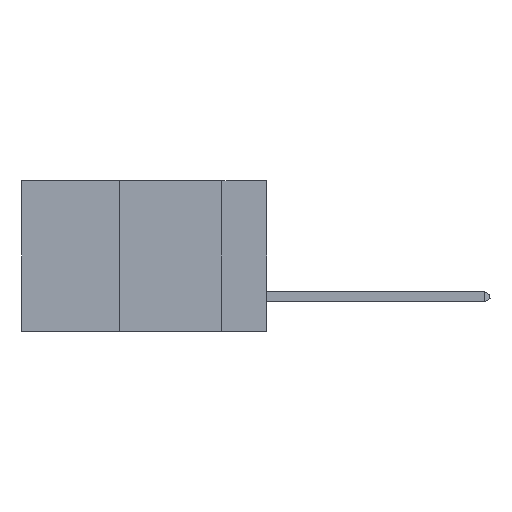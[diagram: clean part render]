
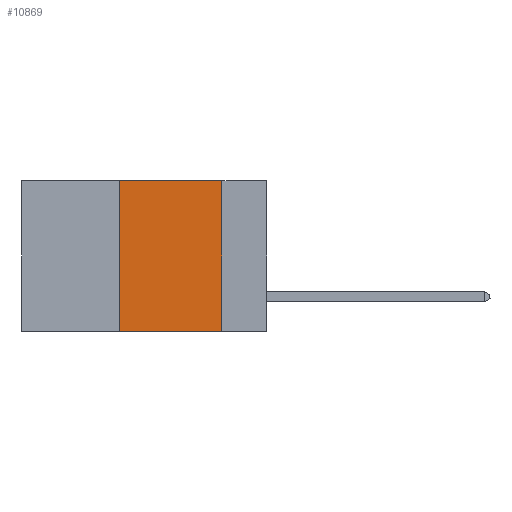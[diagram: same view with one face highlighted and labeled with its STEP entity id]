
A CAD part, left-side view. The second image highlights one B-rep face of the part: STEP entity #10869.
In plain terms, the highlighted planar face has unit normal (-1, 0, 0).
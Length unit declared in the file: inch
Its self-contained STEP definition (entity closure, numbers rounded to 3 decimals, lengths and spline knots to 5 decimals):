
#1000 = CARTESIAN_POINT ( 'NONE',  ( 0., 0.11, 0. ) ) ;
#1123 = CARTESIAN_POINT ( 'NONE',  ( 0., 0.11, -0.37 ) ) ;
#1631 = VERTEX_POINT ( 'NONE', #13952 ) ;
#2370 = DIRECTION ( 'NONE',  ( 0., 0., -1. ) ) ;
#3438 = ORIENTED_EDGE ( 'NONE', *, *, #17596, .F. ) ;
#3608 = AXIS2_PLACEMENT_3D ( 'NONE', #14501, #11351, #2370 ) ;
#3938 = LINE ( 'NONE', #7769, #11267 ) ;
#4342 = DIRECTION ( 'NONE',  ( 0., -1., 0. ) ) ;
#5901 = EDGE_CURVE ( 'NONE', #10032, #9966, #3938, .T. ) ;
#6031 = EDGE_CURVE ( 'NONE', #17533, #10032, #12198, .T. ) ;
#6118 = EDGE_CURVE ( 'NONE', #1631, #9966, #13802, .T. ) ;
#6518 = VECTOR ( 'NONE', #4342, 39.37008 ) ;
#6601 = EDGE_LOOP ( 'NONE', ( #13340, #18307, #3438, #7442 ) ) ;
#7442 = ORIENTED_EDGE ( 'NONE', *, *, #6118, .T. ) ;
#7603 = CARTESIAN_POINT ( 'NONE',  ( 0., 0.6, -0.37 ) ) ;
#7769 = CARTESIAN_POINT ( 'NONE',  ( 0., 0.11, 0. ) ) ;
#8772 = CARTESIAN_POINT ( 'NONE',  ( 0., 0.36, 0. ) ) ;
#9017 = LINE ( 'NONE', #17232, #15106 ) ;
#9966 = VERTEX_POINT ( 'NONE', #1123 ) ;
#10032 = VERTEX_POINT ( 'NONE', #1000 ) ;
#10869 = ADVANCED_FACE ( 'NONE', ( #18545 ), #12900, .F. ) ;
#11267 = VECTOR ( 'NONE', #13776, 39.37008 ) ;
#11351 = DIRECTION ( 'NONE',  ( 1., 0., 0. ) ) ;
#12198 = LINE ( 'NONE', #14618, #19172 ) ;
#12900 = PLANE ( 'NONE',  #3608 ) ;
#13071 = DIRECTION ( 'NONE',  ( 0., -1., 0. ) ) ;
#13340 = ORIENTED_EDGE ( 'NONE', *, *, #5901, .F. ) ;
#13776 = DIRECTION ( 'NONE',  ( 0., 0., -1. ) ) ;
#13802 = LINE ( 'NONE', #7603, #6518 ) ;
#13952 = CARTESIAN_POINT ( 'NONE',  ( 0., 0.36, -0.37 ) ) ;
#14501 = CARTESIAN_POINT ( 'NONE',  ( 0., 0.6, 0. ) ) ;
#14618 = CARTESIAN_POINT ( 'NONE',  ( 0., 0.6, 0. ) ) ;
#15106 = VECTOR ( 'NONE', #17358, 39.37008 ) ;
#17232 = CARTESIAN_POINT ( 'NONE',  ( 0., 0.36, 0. ) ) ;
#17358 = DIRECTION ( 'NONE',  ( 0., 0., 1. ) ) ;
#17533 = VERTEX_POINT ( 'NONE', #8772 ) ;
#17596 = EDGE_CURVE ( 'NONE', #1631, #17533, #9017, .T. ) ;
#18307 = ORIENTED_EDGE ( 'NONE', *, *, #6031, .F. ) ;
#18545 = FACE_OUTER_BOUND ( 'NONE', #6601, .T. ) ;
#19172 = VECTOR ( 'NONE', #13071, 39.37008 ) ;
